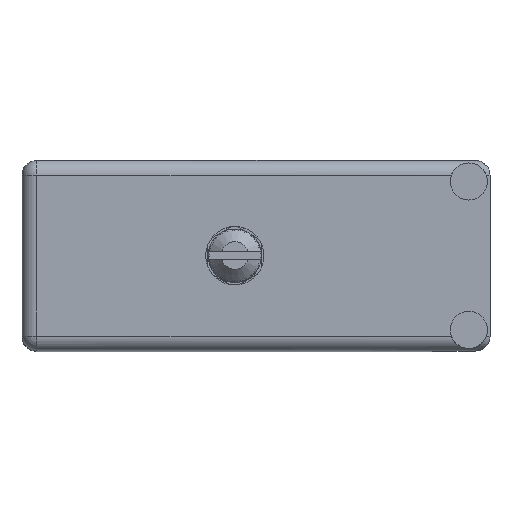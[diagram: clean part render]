
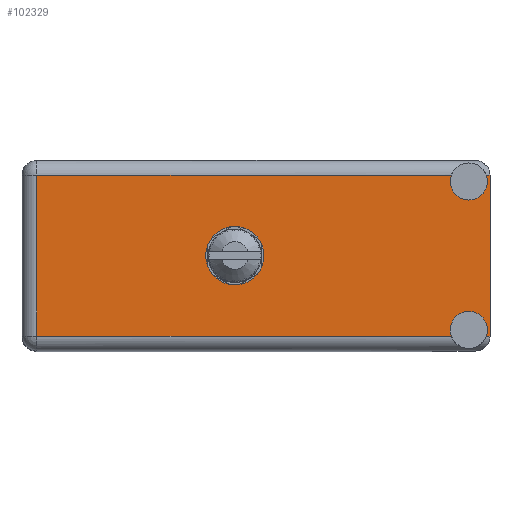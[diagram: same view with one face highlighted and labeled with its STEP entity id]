
A CAD part, top view. The second image highlights one B-rep face of the part: STEP entity #102329.
In plain terms, the highlighted face is planar.
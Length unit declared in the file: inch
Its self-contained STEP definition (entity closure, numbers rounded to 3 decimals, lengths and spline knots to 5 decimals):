
#152 = ORIENTED_EDGE ( 'NONE', *, *, #46128, .F. ) ;
#1571 = EDGE_CURVE ( 'NONE', #81569, #2600, #40604, .T. ) ;
#2600 = VERTEX_POINT ( 'NONE', #23013 ) ;
#2703 = CIRCLE ( 'NONE', #9360, 0.0875 ) ;
#4675 = CARTESIAN_POINT ( 'NONE',  ( 0., 1.566, -0.829 ) ) ;
#4712 = ORIENTED_EDGE ( 'NONE', *, *, #12731, .F. ) ;
#5198 = DIRECTION ( 'NONE',  ( -1., 0., 0. ) ) ;
#6241 = CARTESIAN_POINT ( 'NONE',  ( 1.004, 1.566, -0.587 ) ) ;
#6954 = DIRECTION ( 'NONE',  ( 0., 0., 1. ) ) ;
#7670 = AXIS2_PLACEMENT_3D ( 'NONE', #86704, #95653, #79298 ) ;
#7886 = CARTESIAN_POINT ( 'NONE',  ( 1.004, 1.566, -0.4495 ) ) ;
#9298 = CIRCLE ( 'NONE', #7670, 0.0875 ) ;
#9360 = AXIS2_PLACEMENT_3D ( 'NONE', #42373, #41334, #49264 ) ;
#9600 = VERTEX_POINT ( 'NONE', #14227 ) ;
#10974 = EDGE_CURVE ( 'NONE', #9600, #82319, #70606, .T. ) ;
#11360 = ORIENTED_EDGE ( 'NONE', *, *, #10974, .T. ) ;
#12646 = DIRECTION ( 'NONE',  ( 0., 1., 0. ) ) ;
#12731 = EDGE_CURVE ( 'NONE', #36263, #82319, #50161, .T. ) ;
#13051 = LINE ( 'NONE', #4675, #55724 ) ;
#14227 = CARTESIAN_POINT ( 'NONE',  ( 0.07, 1.566, -0.07 ) ) ;
#14994 = EDGE_CURVE ( 'NONE', #103487, #71185, #80742, .T. ) ;
#15103 = VECTOR ( 'NONE', #104062, 39.37008 ) ;
#15545 = EDGE_CURVE ( 'NONE', #81569, #103866, #49708, .T. ) ;
#18287 = CARTESIAN_POINT ( 'NONE',  ( 2.02562, 1.566, -0.07 ) ) ;
#18743 = ORIENTED_EDGE ( 'NONE', *, *, #1571, .T. ) ;
#21550 = CARTESIAN_POINT ( 'NONE',  ( 2.208, 1.566, -0.07 ) ) ;
#21789 = LINE ( 'NONE', #93554, #71810 ) ;
#22682 = EDGE_CURVE ( 'NONE', #64500, #74561, #2703, .T. ) ;
#23013 = CARTESIAN_POINT ( 'NONE',  ( 2.19038, 1.566, -0.829 ) ) ;
#23295 = DIRECTION ( 'NONE',  ( 0., 0., 1. ) ) ;
#23677 = AXIS2_PLACEMENT_3D ( 'NONE', #23815, #80277, #23295 ) ;
#23815 = CARTESIAN_POINT ( 'NONE',  ( 0., 1.566, -0.899 ) ) ;
#26066 = CIRCLE ( 'NONE', #69846, 0.1375 ) ;
#27603 = VECTOR ( 'NONE', #41619, 39.37008 ) ;
#31525 = VECTOR ( 'NONE', #92966, 39.37008 ) ;
#31998 = CARTESIAN_POINT ( 'NONE',  ( 2.19038, 1.566, -0.07 ) ) ;
#34441 = CARTESIAN_POINT ( 'NONE',  ( 0.07, 1.566, -0.829 ) ) ;
#36263 = VERTEX_POINT ( 'NONE', #81946 ) ;
#36533 = LINE ( 'NONE', #68714, #31525 ) ;
#38422 = DIRECTION ( 'NONE',  ( 0., 1., 0. ) ) ;
#38908 = ORIENTED_EDGE ( 'NONE', *, *, #15545, .F. ) ;
#39104 = DIRECTION ( 'NONE',  ( 0., 0., 1. ) ) ;
#40090 = AXIS2_PLACEMENT_3D ( 'NONE', #45323, #12646, #44796 ) ;
#40604 = LINE ( 'NONE', #65892, #27603 ) ;
#40664 = CARTESIAN_POINT ( 'NONE',  ( 2.108, 1.566, -0.0995 ) ) ;
#41334 = DIRECTION ( 'NONE',  ( 0., 1., 0. ) ) ;
#41619 = DIRECTION ( 'NONE',  ( -1., 0., 0. ) ) ;
#42373 = CARTESIAN_POINT ( 'NONE',  ( 2.108, 1.566, -0.7995 ) ) ;
#44796 = DIRECTION ( 'NONE',  ( 0., 0., 1. ) ) ;
#45323 = CARTESIAN_POINT ( 'NONE',  ( 2.108, 1.566, -0.7995 ) ) ;
#46128 = EDGE_CURVE ( 'NONE', #71185, #103487, #26066, .T. ) ;
#48166 = CARTESIAN_POINT ( 'NONE',  ( 2.208, 1.566, 0. ) ) ;
#48658 = EDGE_CURVE ( 'NONE', #98159, #9600, #21789, .T. ) ;
#49264 = DIRECTION ( 'NONE',  ( 0., 0., 1. ) ) ;
#49383 = ORIENTED_EDGE ( 'NONE', *, *, #51598, .T. ) ;
#49708 = LINE ( 'NONE', #48166, #15103 ) ;
#50161 = CIRCLE ( 'NONE', #65386, 0.0875 ) ;
#51598 = EDGE_CURVE ( 'NONE', #64500, #98159, #13051, .T. ) ;
#51818 = CIRCLE ( 'NONE', #40090, 0.0875 ) ;
#52423 = DIRECTION ( 'NONE',  ( 0., 0., 1. ) ) ;
#52503 = ORIENTED_EDGE ( 'NONE', *, *, #48658, .T. ) ;
#55724 = VECTOR ( 'NONE', #5198, 39.37008 ) ;
#55762 = ORIENTED_EDGE ( 'NONE', *, *, #94666, .T. ) ;
#55858 = CARTESIAN_POINT ( 'NONE',  ( 2.02562, 1.566, -0.829 ) ) ;
#56970 = DIRECTION ( 'NONE',  ( 0., 1., 0. ) ) ;
#58698 = EDGE_CURVE ( 'NONE', #74561, #2600, #51818, .T. ) ;
#58821 = AXIS2_PLACEMENT_3D ( 'NONE', #63332, #56970, #6954 ) ;
#63332 = CARTESIAN_POINT ( 'NONE',  ( 1.004, 1.566, -0.4495 ) ) ;
#63941 = FACE_OUTER_BOUND ( 'NONE', #85741, .T. ) ;
#64500 = VERTEX_POINT ( 'NONE', #55858 ) ;
#65386 = AXIS2_PLACEMENT_3D ( 'NONE', #40664, #72826, #39104 ) ;
#65892 = CARTESIAN_POINT ( 'NONE',  ( 0., 1.566, -0.829 ) ) ;
#67441 = ORIENTED_EDGE ( 'NONE', *, *, #22682, .F. ) ;
#68714 = CARTESIAN_POINT ( 'NONE',  ( 2.208, 1.566, -0.07 ) ) ;
#69291 = ORIENTED_EDGE ( 'NONE', *, *, #14994, .F. ) ;
#69846 = AXIS2_PLACEMENT_3D ( 'NONE', #7886, #38422, #96435 ) ;
#69913 = CARTESIAN_POINT ( 'NONE',  ( 2.108, 1.566, -0.712 ) ) ;
#70606 = LINE ( 'NONE', #21550, #98112 ) ;
#71185 = VERTEX_POINT ( 'NONE', #6241 ) ;
#71810 = VECTOR ( 'NONE', #52423, 39.37008 ) ;
#72826 = DIRECTION ( 'NONE',  ( 0., 1., 0. ) ) ;
#74561 = VERTEX_POINT ( 'NONE', #69913 ) ;
#76064 = VERTEX_POINT ( 'NONE', #31998 ) ;
#79298 = DIRECTION ( 'NONE',  ( 0., 0., 1. ) ) ;
#80092 = EDGE_CURVE ( 'NONE', #76064, #36263, #9298, .T. ) ;
#80231 = CARTESIAN_POINT ( 'NONE',  ( 2.208, 1.566, -0.829 ) ) ;
#80277 = DIRECTION ( 'NONE',  ( 0., 1., 0. ) ) ;
#80439 = EDGE_LOOP ( 'NONE', ( #69291, #152 ) ) ;
#80676 = ORIENTED_EDGE ( 'NONE', *, *, #80092, .F. ) ;
#80742 = CIRCLE ( 'NONE', #58821, 0.1375 ) ;
#81569 = VERTEX_POINT ( 'NONE', #80231 ) ;
#81946 = CARTESIAN_POINT ( 'NONE',  ( 2.108, 1.566, -0.187 ) ) ;
#82319 = VERTEX_POINT ( 'NONE', #18287 ) ;
#85741 = EDGE_LOOP ( 'NONE', ( #11360, #4712, #80676, #55762, #38908, #18743, #96507, #67441, #49383, #52503 ) ) ;
#85916 = DIRECTION ( 'NONE',  ( 1., 0., 0. ) ) ;
#86704 = CARTESIAN_POINT ( 'NONE',  ( 2.108, 1.566, -0.0995 ) ) ;
#87385 = CARTESIAN_POINT ( 'NONE',  ( 1.004, 1.566, -0.312 ) ) ;
#92966 = DIRECTION ( 'NONE',  ( 1., 0., 0. ) ) ;
#93554 = CARTESIAN_POINT ( 'NONE',  ( 0.07, 1.566, -0.899 ) ) ;
#94666 = EDGE_CURVE ( 'NONE', #76064, #103866, #36533, .T. ) ;
#95586 = FACE_BOUND ( 'NONE', #80439, .T. ) ;
#95653 = DIRECTION ( 'NONE',  ( 0., 1., 0. ) ) ;
#96105 = PLANE ( 'NONE',  #23677 ) ;
#96435 = DIRECTION ( 'NONE',  ( 0., 0., 1. ) ) ;
#96507 = ORIENTED_EDGE ( 'NONE', *, *, #58698, .F. ) ;
#98112 = VECTOR ( 'NONE', #85916, 39.37008 ) ;
#98159 = VERTEX_POINT ( 'NONE', #34441 ) ;
#101901 = CARTESIAN_POINT ( 'NONE',  ( 2.208, 1.566, -0.07 ) ) ;
#102329 = ADVANCED_FACE ( 'NONE', ( #95586, #63941 ), #96105, .T. ) ;
#103487 = VERTEX_POINT ( 'NONE', #87385 ) ;
#103866 = VERTEX_POINT ( 'NONE', #101901 ) ;
#104062 = DIRECTION ( 'NONE',  ( 0., 0., 1. ) ) ;
